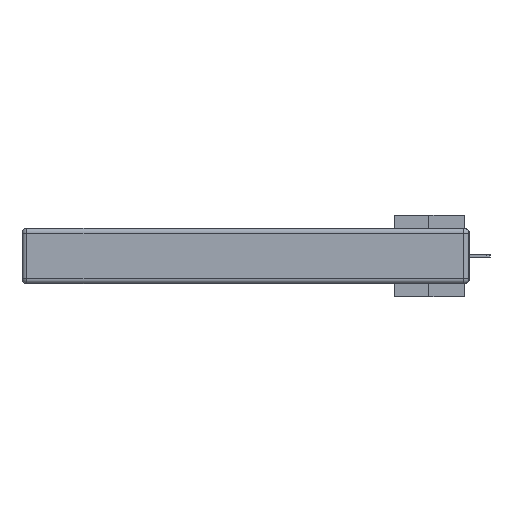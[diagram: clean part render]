
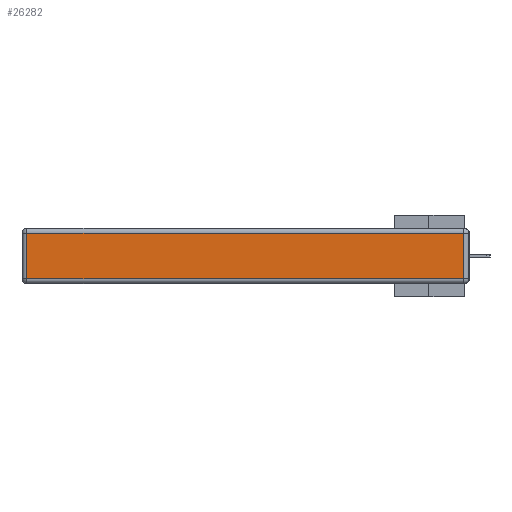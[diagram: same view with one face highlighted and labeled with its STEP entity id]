
A CAD part, left-side view. The second image highlights one B-rep face of the part: STEP entity #26282.
In plain terms, the highlighted planar face has unit normal (-1, 0, 0).
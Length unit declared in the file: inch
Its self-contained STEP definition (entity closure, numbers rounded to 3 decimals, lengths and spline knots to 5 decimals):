
#848 = FACE_OUTER_BOUND ( 'NONE', #28603, .T. ) ;
#1133 = DIRECTION ( 'NONE',  ( 0., 1., 0. ) ) ;
#1840 = EDGE_CURVE ( 'NONE', #13980, #19352, #12407, .T. ) ;
#2487 = VERTEX_POINT ( 'NONE', #33017 ) ;
#3800 = CARTESIAN_POINT ( 'NONE',  ( 0., 0.03, -0.03 ) ) ;
#4100 = CARTESIAN_POINT ( 'NONE',  ( 0., 2.72, -0.343 ) ) ;
#4511 = CARTESIAN_POINT ( 'NONE',  ( 0., 0.03, -0.343 ) ) ;
#5396 = LINE ( 'NONE', #4100, #11963 ) ;
#6171 = CARTESIAN_POINT ( 'NONE',  ( 0., 2.72, -0.313 ) ) ;
#7809 = VERTEX_POINT ( 'NONE', #6171 ) ;
#8636 = AXIS2_PLACEMENT_3D ( 'NONE', #21591, #10434, #30066 ) ;
#9974 = VECTOR ( 'NONE', #1133, 39.37008 ) ;
#10123 = DIRECTION ( 'NONE',  ( 0., 0., 1. ) ) ;
#10434 = DIRECTION ( 'NONE',  ( -1., 0., 0. ) ) ;
#11963 = VECTOR ( 'NONE', #18077, 39.37008 ) ;
#12407 = LINE ( 'NONE', #4511, #19891 ) ;
#12448 = ORIENTED_EDGE ( 'NONE', *, *, #13145, .T. ) ;
#13145 = EDGE_CURVE ( 'NONE', #19352, #2487, #26655, .T. ) ;
#13712 = LINE ( 'NONE', #24687, #27743 ) ;
#13980 = VERTEX_POINT ( 'NONE', #21671 ) ;
#17595 = EDGE_CURVE ( 'NONE', #7809, #13980, #13712, .T. ) ;
#18077 = DIRECTION ( 'NONE',  ( 0., 0., -1. ) ) ;
#19352 = VERTEX_POINT ( 'NONE', #3800 ) ;
#19891 = VECTOR ( 'NONE', #10123, 39.37008 ) ;
#20757 = CARTESIAN_POINT ( 'NONE',  ( 0., 2.75, -0.03 ) ) ;
#21591 = CARTESIAN_POINT ( 'NONE',  ( 0., 0., -0.343 ) ) ;
#21671 = CARTESIAN_POINT ( 'NONE',  ( 0., 0.03, -0.313 ) ) ;
#22281 = ORIENTED_EDGE ( 'NONE', *, *, #1840, .T. ) ;
#24687 = CARTESIAN_POINT ( 'NONE',  ( 0., 0., -0.313 ) ) ;
#26282 = ADVANCED_FACE ( 'NONE', ( #848 ), #27241, .T. ) ;
#26655 = LINE ( 'NONE', #20757, #9974 ) ;
#27241 = PLANE ( 'NONE',  #8636 ) ;
#27743 = VECTOR ( 'NONE', #33036, 39.37008 ) ;
#28603 = EDGE_LOOP ( 'NONE', ( #34081, #22281, #12448, #31124 ) ) ;
#30066 = DIRECTION ( 'NONE',  ( 0., 0., 1. ) ) ;
#30827 = EDGE_CURVE ( 'NONE', #2487, #7809, #5396, .T. ) ;
#31124 = ORIENTED_EDGE ( 'NONE', *, *, #30827, .T. ) ;
#33017 = CARTESIAN_POINT ( 'NONE',  ( 0., 2.72, -0.03 ) ) ;
#33036 = DIRECTION ( 'NONE',  ( 0., -1., 0. ) ) ;
#34081 = ORIENTED_EDGE ( 'NONE', *, *, #17595, .T. ) ;
